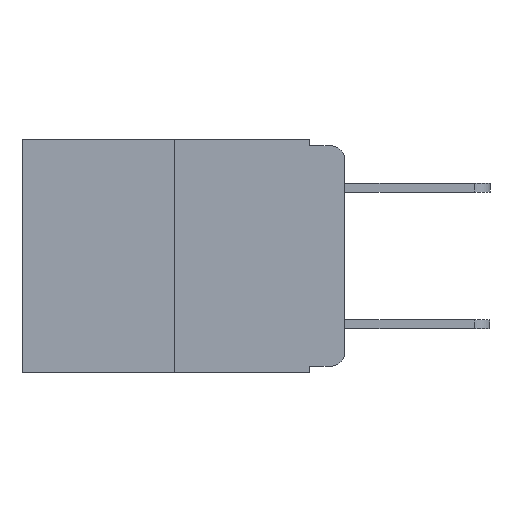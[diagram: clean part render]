
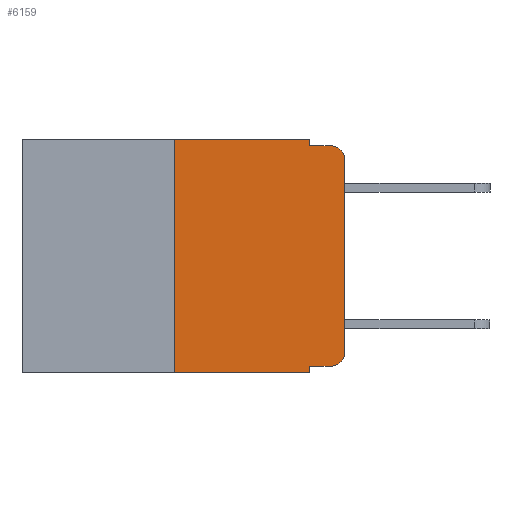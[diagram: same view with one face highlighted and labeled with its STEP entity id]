
A CAD part, left-side view. The second image highlights one B-rep face of the part: STEP entity #6159.
In plain terms, the highlighted planar face has unit normal (-1, 0, 0).
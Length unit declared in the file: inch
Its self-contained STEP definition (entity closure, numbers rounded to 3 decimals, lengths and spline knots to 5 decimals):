
#92 = VERTEX_POINT ( 'NONE', #501 ) ;
#296 = VECTOR ( 'NONE', #6070, 39.37008 ) ;
#501 = CARTESIAN_POINT ( 'NONE',  ( 0., 0., -0.313 ) ) ;
#513 = EDGE_CURVE ( 'NONE', #1980, #1772, #2778, .T. ) ;
#763 = CARTESIAN_POINT ( 'NONE',  ( 0., 0.473, -0.343 ) ) ;
#874 = DIRECTION ( 'NONE',  ( 0., -1., 0. ) ) ;
#1549 = VERTEX_POINT ( 'NONE', #4547 ) ;
#1644 = CARTESIAN_POINT ( 'NONE',  ( 0., 0.051, 0. ) ) ;
#1772 = VERTEX_POINT ( 'NONE', #4034 ) ;
#1980 = VERTEX_POINT ( 'NONE', #9017 ) ;
#2042 = CIRCLE ( 'NONE', #7551, 0.02 ) ;
#2188 = CARTESIAN_POINT ( 'NONE',  ( 0., 0., 0. ) ) ;
#2297 = VECTOR ( 'NONE', #3236, 39.37008 ) ;
#2435 = EDGE_CURVE ( 'NONE', #1549, #92, #8843, .T. ) ;
#2778 = LINE ( 'NONE', #7998, #296 ) ;
#2802 = EDGE_CURVE ( 'NONE', #4008, #4567, #7813, .T. ) ;
#3086 = DIRECTION ( 'NONE',  ( 0., 0., 1. ) ) ;
#3211 = EDGE_CURVE ( 'NONE', #3270, #8081, #8447, .T. ) ;
#3236 = DIRECTION ( 'NONE',  ( 0., 0., -1. ) ) ;
#3270 = VERTEX_POINT ( 'NONE', #7541 ) ;
#3282 = EDGE_CURVE ( 'NONE', #4008, #3270, #6104, .T. ) ;
#3385 = PLANE ( 'NONE',  #7916 ) ;
#3521 = EDGE_CURVE ( 'NONE', #8366, #1549, #6768, .T. ) ;
#3527 = EDGE_CURVE ( 'NONE', #92, #3671, #4779, .T. ) ;
#3574 = EDGE_CURVE ( 'NONE', #3671, #1772, #2042, .T. ) ;
#3671 = VERTEX_POINT ( 'NONE', #6326 ) ;
#3787 = EDGE_CURVE ( 'NONE', #8081, #1980, #6573, .T. ) ;
#3919 = DIRECTION ( 'NONE',  ( -1., 0., 0. ) ) ;
#4004 = VECTOR ( 'NONE', #874, 39.37008 ) ;
#4008 = VERTEX_POINT ( 'NONE', #5890 ) ;
#4034 = CARTESIAN_POINT ( 'NONE',  ( 0., 0.02, -0.01 ) ) ;
#4159 = CARTESIAN_POINT ( 'NONE',  ( 0., 0.473, 0. ) ) ;
#4206 = CARTESIAN_POINT ( 'NONE',  ( 0., 0.25, 0. ) ) ;
#4307 = EDGE_CURVE ( 'NONE', #8366, #4567, #6565, .T. ) ;
#4547 = CARTESIAN_POINT ( 'NONE',  ( 0., 0.02, -0.333 ) ) ;
#4567 = VERTEX_POINT ( 'NONE', #7211 ) ;
#4579 = ORIENTED_EDGE ( 'NONE', *, *, #3527, .T. ) ;
#4632 = ORIENTED_EDGE ( 'NONE', *, *, #3574, .T. ) ;
#4643 = VECTOR ( 'NONE', #8085, 39.37008 ) ;
#4650 = DIRECTION ( 'NONE',  ( 0., -1., 0. ) ) ;
#4670 = ORIENTED_EDGE ( 'NONE', *, *, #513, .F. ) ;
#4768 = VECTOR ( 'NONE', #8234, 39.37008 ) ;
#4779 = LINE ( 'NONE', #2188, #8010 ) ;
#4824 = CARTESIAN_POINT ( 'NONE',  ( 0., 0.051, 0. ) ) ;
#4965 = DIRECTION ( 'NONE',  ( 0., 0., -1. ) ) ;
#5004 = VECTOR ( 'NONE', #4650, 39.37008 ) ;
#5062 = ORIENTED_EDGE ( 'NONE', *, *, #3787, .F. ) ;
#5240 = ORIENTED_EDGE ( 'NONE', *, *, #3211, .F. ) ;
#5306 = ORIENTED_EDGE ( 'NONE', *, *, #3282, .F. ) ;
#5443 = ORIENTED_EDGE ( 'NONE', *, *, #2802, .T. ) ;
#5489 = ORIENTED_EDGE ( 'NONE', *, *, #4307, .F. ) ;
#5752 = ORIENTED_EDGE ( 'NONE', *, *, #3521, .T. ) ;
#5792 = CARTESIAN_POINT ( 'NONE',  ( 0., 0.051, -0.333 ) ) ;
#5890 = CARTESIAN_POINT ( 'NONE',  ( 0., 0.25, -0.343 ) ) ;
#5989 = ORIENTED_EDGE ( 'NONE', *, *, #2435, .T. ) ;
#6068 = CARTESIAN_POINT ( 'NONE',  ( 0., 0.051, -0.333 ) ) ;
#6070 = DIRECTION ( 'NONE',  ( 0., -1., 0. ) ) ;
#6104 = LINE ( 'NONE', #4206, #7256 ) ;
#6159 = ADVANCED_FACE ( 'NONE', ( #6656 ), #3385, .F. ) ;
#6326 = CARTESIAN_POINT ( 'NONE',  ( 0., 0., -0.03 ) ) ;
#6565 = LINE ( 'NONE', #4824, #2297 ) ;
#6573 = LINE ( 'NONE', #8214, #4768 ) ;
#6656 = FACE_OUTER_BOUND ( 'NONE', #9129, .T. ) ;
#6768 = LINE ( 'NONE', #6068, #5004 ) ;
#7133 = CARTESIAN_POINT ( 'NONE',  ( 0., 0.02, -0.313 ) ) ;
#7211 = CARTESIAN_POINT ( 'NONE',  ( 0., 0.051, -0.343 ) ) ;
#7256 = VECTOR ( 'NONE', #9318, 39.37008 ) ;
#7285 = DIRECTION ( 'NONE',  ( 0., 0., -1. ) ) ;
#7313 = DIRECTION ( 'NONE',  ( -1., 0., 0. ) ) ;
#7541 = CARTESIAN_POINT ( 'NONE',  ( 0., 0.25, 0. ) ) ;
#7551 = AXIS2_PLACEMENT_3D ( 'NONE', #7978, #3919, #8561 ) ;
#7813 = LINE ( 'NONE', #763, #4004 ) ;
#7916 = AXIS2_PLACEMENT_3D ( 'NONE', #4159, #8738, #4965 ) ;
#7978 = CARTESIAN_POINT ( 'NONE',  ( 0., 0.02, -0.03 ) ) ;
#7998 = CARTESIAN_POINT ( 'NONE',  ( 0., 0.051, -0.01 ) ) ;
#8010 = VECTOR ( 'NONE', #3086, 39.37008 ) ;
#8081 = VERTEX_POINT ( 'NONE', #1644 ) ;
#8085 = DIRECTION ( 'NONE',  ( 0., -1., 0. ) ) ;
#8214 = CARTESIAN_POINT ( 'NONE',  ( 0., 0.051, 0. ) ) ;
#8234 = DIRECTION ( 'NONE',  ( 0., 0., -1. ) ) ;
#8360 = AXIS2_PLACEMENT_3D ( 'NONE', #7133, #7313, #7285 ) ;
#8366 = VERTEX_POINT ( 'NONE', #5792 ) ;
#8447 = LINE ( 'NONE', #8674, #4643 ) ;
#8561 = DIRECTION ( 'NONE',  ( 0., 0., -1. ) ) ;
#8674 = CARTESIAN_POINT ( 'NONE',  ( 0., 0.473, 0. ) ) ;
#8738 = DIRECTION ( 'NONE',  ( 1., 0., 0. ) ) ;
#8843 = CIRCLE ( 'NONE', #8360, 0.02 ) ;
#9017 = CARTESIAN_POINT ( 'NONE',  ( 0., 0.051, -0.01 ) ) ;
#9129 = EDGE_LOOP ( 'NONE', ( #4579, #4632, #4670, #5062, #5240, #5306, #5443, #5489, #5752, #5989 ) ) ;
#9318 = DIRECTION ( 'NONE',  ( 0., 0., 1. ) ) ;
